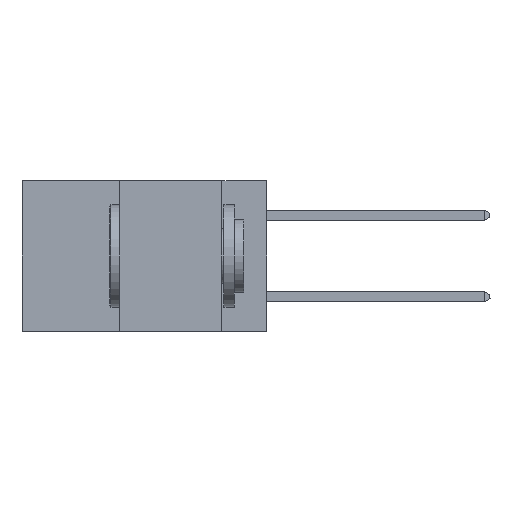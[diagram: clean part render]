
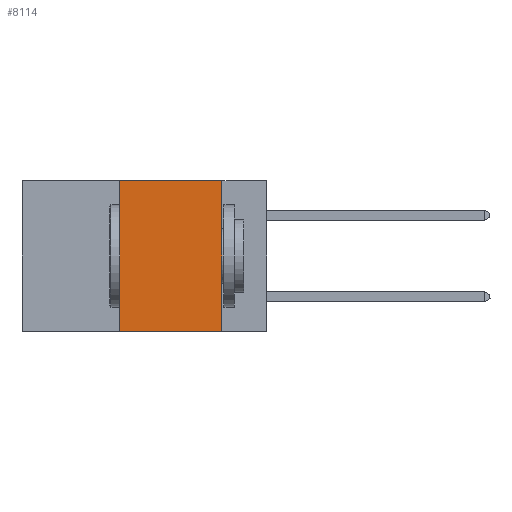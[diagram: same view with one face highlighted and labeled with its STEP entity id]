
A CAD part, left-side view. The second image highlights one B-rep face of the part: STEP entity #8114.
In plain terms, the highlighted planar face has unit normal (-1, 0, 0).
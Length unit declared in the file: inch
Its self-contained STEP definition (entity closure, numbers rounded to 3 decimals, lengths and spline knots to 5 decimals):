
#1280 = VERTEX_POINT ( 'NONE', #3165 ) ;
#1551 = ORIENTED_EDGE ( 'NONE', *, *, #4003, .F. ) ;
#3165 = CARTESIAN_POINT ( 'NONE',  ( 0., 0.36, -0.37 ) ) ;
#3211 = EDGE_CURVE ( 'NONE', #1280, #14616, #45458, .T. ) ;
#4003 = EDGE_CURVE ( 'NONE', #6875, #14616, #36103, .T. ) ;
#4158 = EDGE_CURVE ( 'NONE', #1280, #5294, #34468, .T. ) ;
#5294 = VERTEX_POINT ( 'NONE', #16382 ) ;
#6875 = VERTEX_POINT ( 'NONE', #45730 ) ;
#8114 = ADVANCED_FACE ( 'NONE', ( #43403 ), #14364, .F. ) ;
#8806 = VECTOR ( 'NONE', #29328, 39.37008 ) ;
#13036 = CARTESIAN_POINT ( 'NONE',  ( 0., 0.6, 0. ) ) ;
#13821 = DIRECTION ( 'NONE',  ( 0., 0., -1. ) ) ;
#14364 = PLANE ( 'NONE',  #16465 ) ;
#14616 = VERTEX_POINT ( 'NONE', #20481 ) ;
#16095 = EDGE_LOOP ( 'NONE', ( #1551, #43880, #19085, #42456 ) ) ;
#16382 = CARTESIAN_POINT ( 'NONE',  ( 0., 0.36, 0. ) ) ;
#16465 = AXIS2_PLACEMENT_3D ( 'NONE', #13036, #31592, #31809 ) ;
#19085 = ORIENTED_EDGE ( 'NONE', *, *, #4158, .F. ) ;
#20481 = CARTESIAN_POINT ( 'NONE',  ( 0., 0.11, -0.37 ) ) ;
#23908 = CARTESIAN_POINT ( 'NONE',  ( 0., 0.6, -0.37 ) ) ;
#24969 = CARTESIAN_POINT ( 'NONE',  ( 0., 0.11, 0. ) ) ;
#25157 = CARTESIAN_POINT ( 'NONE',  ( 0., 0.36, 0. ) ) ;
#25825 = CARTESIAN_POINT ( 'NONE',  ( 0., 0.6, 0. ) ) ;
#26362 = DIRECTION ( 'NONE',  ( 0., 0., 1. ) ) ;
#29328 = DIRECTION ( 'NONE',  ( 0., -1., 0. ) ) ;
#31592 = DIRECTION ( 'NONE',  ( 1., 0., 0. ) ) ;
#31809 = DIRECTION ( 'NONE',  ( 0., 0., -1. ) ) ;
#34349 = VECTOR ( 'NONE', #26362, 39.37008 ) ;
#34468 = LINE ( 'NONE', #25157, #34349 ) ;
#35773 = VECTOR ( 'NONE', #13821, 39.37008 ) ;
#36103 = LINE ( 'NONE', #24969, #35773 ) ;
#38911 = EDGE_CURVE ( 'NONE', #5294, #6875, #46105, .T. ) ;
#42456 = ORIENTED_EDGE ( 'NONE', *, *, #3211, .T. ) ;
#42701 = DIRECTION ( 'NONE',  ( 0., -1., 0. ) ) ;
#43403 = FACE_OUTER_BOUND ( 'NONE', #16095, .T. ) ;
#43880 = ORIENTED_EDGE ( 'NONE', *, *, #38911, .F. ) ;
#45458 = LINE ( 'NONE', #23908, #45584 ) ;
#45584 = VECTOR ( 'NONE', #42701, 39.37008 ) ;
#45730 = CARTESIAN_POINT ( 'NONE',  ( 0., 0.11, 0. ) ) ;
#46105 = LINE ( 'NONE', #25825, #8806 ) ;
